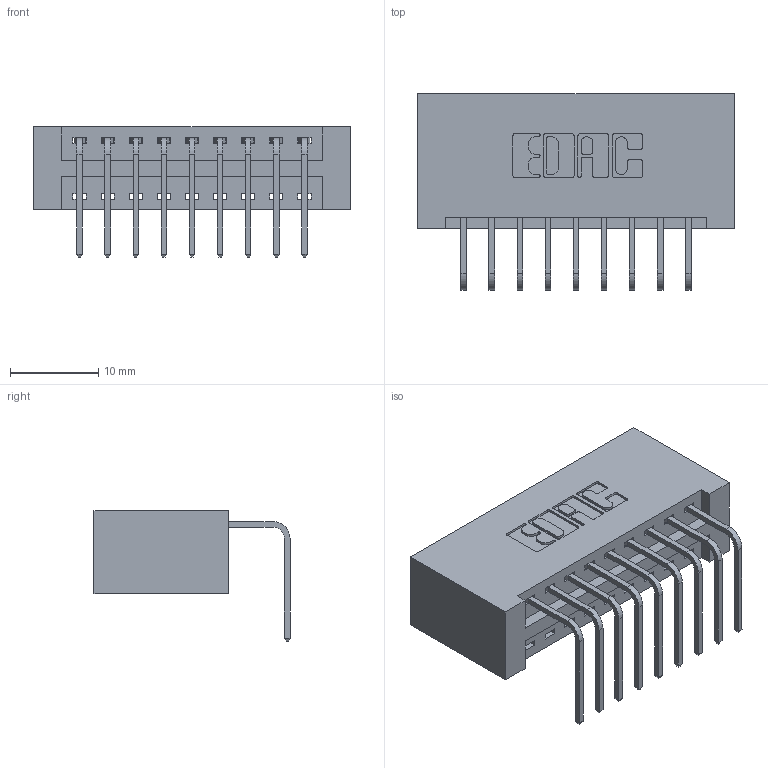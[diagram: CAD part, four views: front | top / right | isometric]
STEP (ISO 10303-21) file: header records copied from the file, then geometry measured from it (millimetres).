
FILE_DESCRIPTION (( 'STEP AP203' ), '1' );
FILE_NAME ('346-009-558-101.STEP', '2018-08-17T05:55:33', ( '' ), ( '' ), 'SwSTEP 2.0', 'SolidWorks 2016', '' );
FILE_SCHEMA (( 'CONFIG_CONTROL_DESIGN' ));
Length unit declared in the file: inch
Products named in the file (3): 346-009-558-101; 346 Part_No Mounting Lugs; 345-292-001_558 Tail - 2
Assembly tree (10 placements, depth 2):
  346-009-558-101
    346 Part_No Mounting Lugs
    345-292-001_558 Tail - 2  x9
Bounding box: 35.81 x 22.16 x 14.73 mm (x, y, z)
Volume: 3780.2 mm3; surface area: 4622.7 mm2
Topology: 10 solids, 10 shells, 654 faces, 1943 edges, 1282 vertices
Faces by surface type: plane 450, cylinder 204
Entity records: 9835 total; most frequent: CARTESIAN_POINT 1703, ORIENTED_EDGE 1646, DIRECTION 1537, EDGE_CURVE 823, LINE 663, VECTOR 663, VERTEX_POINT 546, AXIS2_PLACEMENT_3D 437
